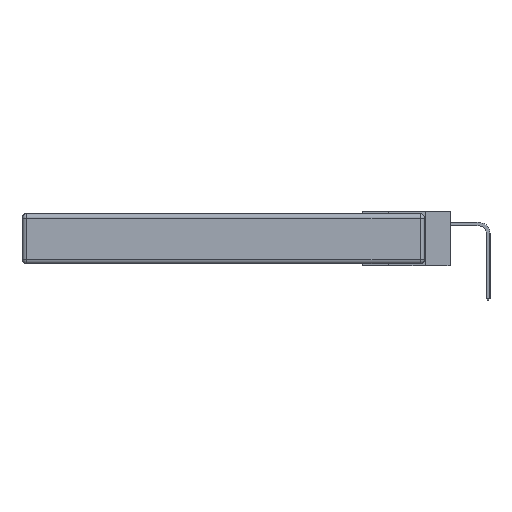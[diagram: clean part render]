
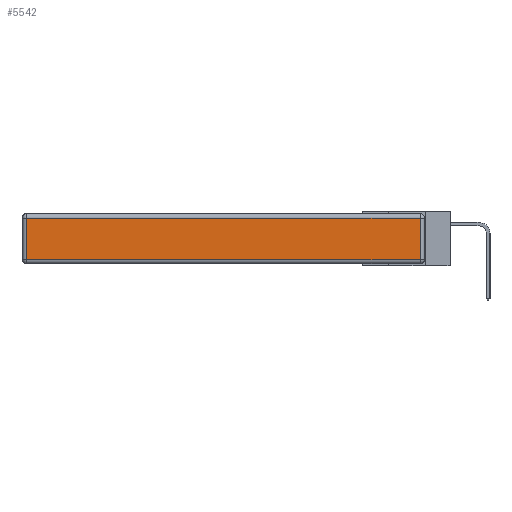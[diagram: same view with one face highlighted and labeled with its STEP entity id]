
A CAD part, left-side view. The second image highlights one B-rep face of the part: STEP entity #5542.
In plain terms, the highlighted planar face has unit normal (-1, 0, 0).
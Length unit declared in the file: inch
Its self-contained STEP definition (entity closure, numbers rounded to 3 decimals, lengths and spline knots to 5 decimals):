
#709 = CARTESIAN_POINT ( 'NONE',  ( 0., 2.72, -0.313 ) ) ;
#1300 = DIRECTION ( 'NONE',  ( -1., 0., 0. ) ) ;
#1706 = DIRECTION ( 'NONE',  ( 0., -1., 0. ) ) ;
#2449 = ORIENTED_EDGE ( 'NONE', *, *, #5759, .T. ) ;
#3249 = CARTESIAN_POINT ( 'NONE',  ( 0., 0., -0.343 ) ) ;
#3841 = VECTOR ( 'NONE', #1706, 39.37008 ) ;
#3871 = CARTESIAN_POINT ( 'NONE',  ( 0., 2.75, -0.03 ) ) ;
#4973 = EDGE_CURVE ( 'NONE', #17123, #11207, #20415, .T. ) ;
#5026 = VERTEX_POINT ( 'NONE', #17981 ) ;
#5542 = ADVANCED_FACE ( 'NONE', ( #14796 ), #12276, .T. ) ;
#5759 = EDGE_CURVE ( 'NONE', #9564, #17123, #9765, .T. ) ;
#6474 = EDGE_CURVE ( 'NONE', #11207, #5026, #13917, .T. ) ;
#6480 = ORIENTED_EDGE ( 'NONE', *, *, #4973, .T. ) ;
#6762 = CARTESIAN_POINT ( 'NONE',  ( 0., 0.03, -0.343 ) ) ;
#7001 = ORIENTED_EDGE ( 'NONE', *, *, #6474, .T. ) ;
#7173 = ORIENTED_EDGE ( 'NONE', *, *, #15720, .T. ) ;
#7197 = AXIS2_PLACEMENT_3D ( 'NONE', #3249, #1300, #20994 ) ;
#7375 = DIRECTION ( 'NONE',  ( 0., 0., 1. ) ) ;
#9564 = VERTEX_POINT ( 'NONE', #709 ) ;
#9765 = LINE ( 'NONE', #19616, #3841 ) ;
#10590 = CARTESIAN_POINT ( 'NONE',  ( 0., 2.72, -0.343 ) ) ;
#11104 = DIRECTION ( 'NONE',  ( 0., 1., 0. ) ) ;
#11207 = VERTEX_POINT ( 'NONE', #13164 ) ;
#11503 = LINE ( 'NONE', #10590, #14848 ) ;
#12276 = PLANE ( 'NONE',  #7197 ) ;
#13164 = CARTESIAN_POINT ( 'NONE',  ( 0., 0.03, -0.03 ) ) ;
#13443 = EDGE_LOOP ( 'NONE', ( #2449, #6480, #7001, #7173 ) ) ;
#13917 = LINE ( 'NONE', #3871, #21147 ) ;
#14796 = FACE_OUTER_BOUND ( 'NONE', #13443, .T. ) ;
#14848 = VECTOR ( 'NONE', #19624, 39.37008 ) ;
#15388 = VECTOR ( 'NONE', #7375, 39.37008 ) ;
#15720 = EDGE_CURVE ( 'NONE', #5026, #9564, #11503, .T. ) ;
#15775 = CARTESIAN_POINT ( 'NONE',  ( 0., 0.03, -0.313 ) ) ;
#17123 = VERTEX_POINT ( 'NONE', #15775 ) ;
#17981 = CARTESIAN_POINT ( 'NONE',  ( 0., 2.72, -0.03 ) ) ;
#19616 = CARTESIAN_POINT ( 'NONE',  ( 0., 0., -0.313 ) ) ;
#19624 = DIRECTION ( 'NONE',  ( 0., 0., -1. ) ) ;
#20415 = LINE ( 'NONE', #6762, #15388 ) ;
#20994 = DIRECTION ( 'NONE',  ( 0., 0., 1. ) ) ;
#21147 = VECTOR ( 'NONE', #11104, 39.37008 ) ;
